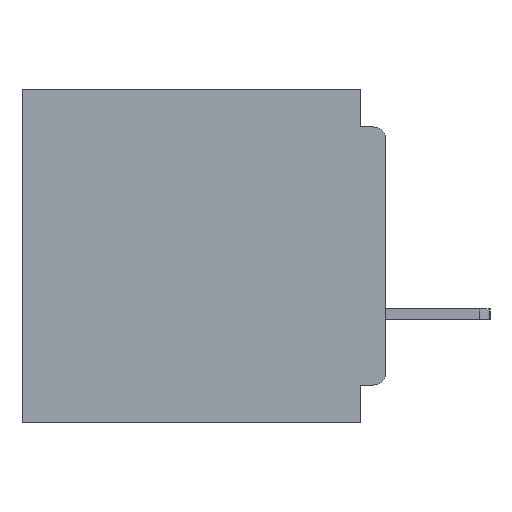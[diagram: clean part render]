
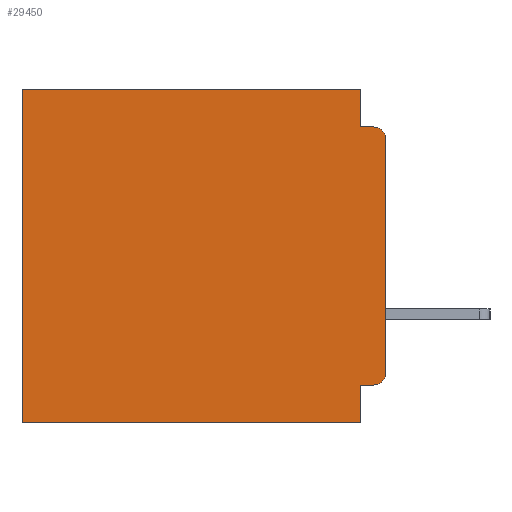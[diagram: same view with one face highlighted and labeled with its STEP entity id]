
A CAD part, left-side view. The second image highlights one B-rep face of the part: STEP entity #29450.
In plain terms, the highlighted planar face has unit normal (-1, 0, 0).
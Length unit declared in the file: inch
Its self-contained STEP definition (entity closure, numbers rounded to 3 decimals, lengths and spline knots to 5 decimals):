
#2325 = CARTESIAN_POINT ( 'NONE',  ( 0.3, 0., 0. ) ) ;
#2356 = DIRECTION ( 'NONE',  ( 0., 1., 0. ) ) ;
#4780 = CARTESIAN_POINT ( 'NONE',  ( 0.3, 0., -0.06 ) ) ;
#6098 = CARTESIAN_POINT ( 'NONE',  ( 0.3, 0.015, -0.06 ) ) ;
#6114 = CARTESIAN_POINT ( 'NONE',  ( 0.3, 0.031, -0.355 ) ) ;
#6577 = CARTESIAN_POINT ( 'NONE',  ( 0.3, 0.015, -0.045 ) ) ;
#7682 = AXIS2_PLACEMENT_3D ( 'NONE', #63610, #43083, #12179 ) ;
#9007 = EDGE_CURVE ( 'NONE', #36479, #42275, #61090, .T. ) ;
#9193 = VECTOR ( 'NONE', #15373, 39.37008 ) ;
#9713 = ORIENTED_EDGE ( 'NONE', *, *, #12913, .F. ) ;
#9930 = VECTOR ( 'NONE', #51360, 39.37008 ) ;
#10506 = LINE ( 'NONE', #59352, #36326 ) ;
#10977 = DIRECTION ( 'NONE',  ( 0., 0., -1. ) ) ;
#11322 = DIRECTION ( 'NONE',  ( 0., 0., -1. ) ) ;
#12051 = ORIENTED_EDGE ( 'NONE', *, *, #52481, .F. ) ;
#12126 = ORIENTED_EDGE ( 'NONE', *, *, #26318, .T. ) ;
#12179 = DIRECTION ( 'NONE',  ( 0., 0., -1. ) ) ;
#12212 = VECTOR ( 'NONE', #17940, 39.37008 ) ;
#12913 = EDGE_CURVE ( 'NONE', #25849, #66262, #51127, .T. ) ;
#13564 = EDGE_CURVE ( 'NONE', #51522, #38943, #24398, .T. ) ;
#14844 = CARTESIAN_POINT ( 'NONE',  ( 0.3, 0.437, 0. ) ) ;
#14900 = AXIS2_PLACEMENT_3D ( 'NONE', #46139, #15226, #51337 ) ;
#15226 = DIRECTION ( 'NONE',  ( -1., 0., 0. ) ) ;
#15373 = DIRECTION ( 'NONE',  ( 0., 0., -1. ) ) ;
#17129 = PLANE ( 'NONE',  #7682 ) ;
#17940 = DIRECTION ( 'NONE',  ( 0., 1., 0. ) ) ;
#18001 = CIRCLE ( 'NONE', #14900, 0.015 ) ;
#18071 = DIRECTION ( 'NONE',  ( 0., 0., -1. ) ) ;
#19013 = CARTESIAN_POINT ( 'NONE',  ( 0.3, 0.031, -0.045 ) ) ;
#20520 = ORIENTED_EDGE ( 'NONE', *, *, #25162, .F. ) ;
#21480 = CARTESIAN_POINT ( 'NONE',  ( 0.3, 0., -0.34 ) ) ;
#22933 = LINE ( 'NONE', #66776, #9193 ) ;
#23555 = EDGE_CURVE ( 'NONE', #66262, #28449, #57834, .T. ) ;
#24398 = CIRCLE ( 'NONE', #28938, 0.015 ) ;
#25162 = EDGE_CURVE ( 'NONE', #58598, #59213, #22933, .T. ) ;
#25849 = VERTEX_POINT ( 'NONE', #62855 ) ;
#26318 = EDGE_CURVE ( 'NONE', #25849, #38873, #18001, .T. ) ;
#28043 = DIRECTION ( 'NONE',  ( 0., 0., -1. ) ) ;
#28045 = CARTESIAN_POINT ( 'NONE',  ( 0.3, 0.031, -0.4 ) ) ;
#28449 = VERTEX_POINT ( 'NONE', #28045 ) ;
#28938 = AXIS2_PLACEMENT_3D ( 'NONE', #6098, #42222, #11322 ) ;
#29155 = ORIENTED_EDGE ( 'NONE', *, *, #13564, .T. ) ;
#29450 = ADVANCED_FACE ( 'NONE', ( #65967 ), #17129, .F. ) ;
#30390 = VECTOR ( 'NONE', #28043, 39.37008 ) ;
#30622 = CARTESIAN_POINT ( 'NONE',  ( 0.3, 0., -0.045 ) ) ;
#30734 = CARTESIAN_POINT ( 'NONE',  ( 0.3, 0.031, 0. ) ) ;
#32684 = EDGE_LOOP ( 'NONE', ( #58111, #29155, #53985, #20520, #51795, #64152, #12051, #41421, #9713, #12126 ) ) ;
#33423 = LINE ( 'NONE', #30622, #45587 ) ;
#35087 = EDGE_CURVE ( 'NONE', #58598, #36479, #55023, .T. ) ;
#36326 = VECTOR ( 'NONE', #18071, 39.37008 ) ;
#36479 = VERTEX_POINT ( 'NONE', #14844 ) ;
#38873 = VERTEX_POINT ( 'NONE', #21480 ) ;
#38943 = VERTEX_POINT ( 'NONE', #6577 ) ;
#39076 = EDGE_CURVE ( 'NONE', #51522, #38873, #10506, .T. ) ;
#41421 = ORIENTED_EDGE ( 'NONE', *, *, #23555, .F. ) ;
#42222 = DIRECTION ( 'NONE',  ( -1., 0., 0. ) ) ;
#42275 = VERTEX_POINT ( 'NONE', #53095 ) ;
#42453 = CARTESIAN_POINT ( 'NONE',  ( 0.3, 0.031, -0.4 ) ) ;
#42733 = VECTOR ( 'NONE', #2356, 39.37008 ) ;
#43083 = DIRECTION ( 'NONE',  ( 1., 0., 0. ) ) ;
#45587 = VECTOR ( 'NONE', #51193, 39.37008 ) ;
#46139 = CARTESIAN_POINT ( 'NONE',  ( 0.3, 0.015, -0.34 ) ) ;
#46157 = CARTESIAN_POINT ( 'NONE',  ( 0.3, 0., -0.355 ) ) ;
#48678 = CARTESIAN_POINT ( 'NONE',  ( 0.3, 0., -0.4 ) ) ;
#51127 = LINE ( 'NONE', #46157, #9930 ) ;
#51193 = DIRECTION ( 'NONE',  ( 0., -1., 0. ) ) ;
#51337 = DIRECTION ( 'NONE',  ( 0., 0., -1. ) ) ;
#51360 = DIRECTION ( 'NONE',  ( 0., 1., 0. ) ) ;
#51522 = VERTEX_POINT ( 'NONE', #4780 ) ;
#51795 = ORIENTED_EDGE ( 'NONE', *, *, #35087, .T. ) ;
#51853 = CARTESIAN_POINT ( 'NONE',  ( 0.3, 0.437, -0.4 ) ) ;
#52481 = EDGE_CURVE ( 'NONE', #28449, #42275, #56453, .T. ) ;
#53095 = CARTESIAN_POINT ( 'NONE',  ( 0.3, 0.437, -0.4 ) ) ;
#53985 = ORIENTED_EDGE ( 'NONE', *, *, #60007, .F. ) ;
#55023 = LINE ( 'NONE', #2325, #12212 ) ;
#56453 = LINE ( 'NONE', #48678, #42733 ) ;
#57834 = LINE ( 'NONE', #42453, #30390 ) ;
#58111 = ORIENTED_EDGE ( 'NONE', *, *, #39076, .F. ) ;
#58598 = VERTEX_POINT ( 'NONE', #30734 ) ;
#59213 = VERTEX_POINT ( 'NONE', #19013 ) ;
#59352 = CARTESIAN_POINT ( 'NONE',  ( 0.3, 0., -0.4 ) ) ;
#59476 = VECTOR ( 'NONE', #10977, 39.37008 ) ;
#60007 = EDGE_CURVE ( 'NONE', #59213, #38943, #33423, .T. ) ;
#61090 = LINE ( 'NONE', #51853, #59476 ) ;
#62855 = CARTESIAN_POINT ( 'NONE',  ( 0.3, 0.015, -0.355 ) ) ;
#63610 = CARTESIAN_POINT ( 'NONE',  ( 0.3, 0., -0.4 ) ) ;
#64152 = ORIENTED_EDGE ( 'NONE', *, *, #9007, .T. ) ;
#65967 = FACE_OUTER_BOUND ( 'NONE', #32684, .T. ) ;
#66262 = VERTEX_POINT ( 'NONE', #6114 ) ;
#66776 = CARTESIAN_POINT ( 'NONE',  ( 0.3, 0.031, 0. ) ) ;
